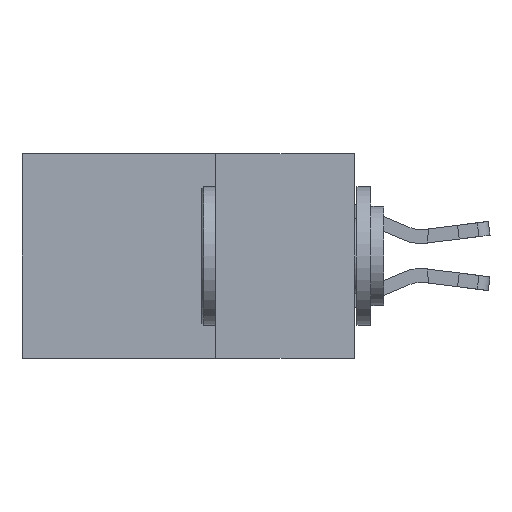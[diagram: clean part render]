
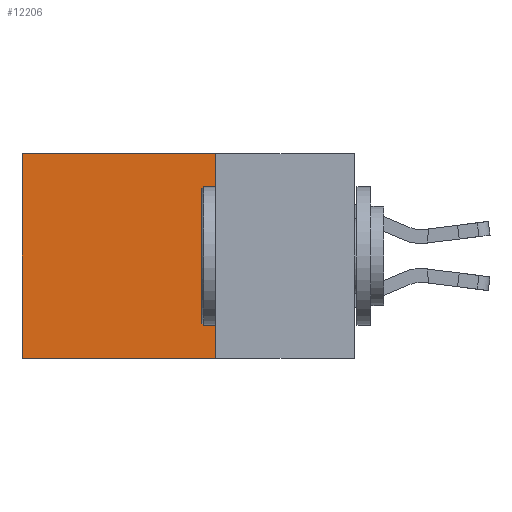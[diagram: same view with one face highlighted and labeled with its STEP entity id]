
A CAD part, left-side view. The second image highlights one B-rep face of the part: STEP entity #12206.
In plain terms, the highlighted planar face has unit normal (-1, 0, 0).
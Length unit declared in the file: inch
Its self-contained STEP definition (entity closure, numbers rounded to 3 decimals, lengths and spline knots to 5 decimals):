
#450 = CARTESIAN_POINT ( 'NONE',  ( 0.298, 0.25, -0.37 ) ) ;
#721 = LINE ( 'NONE', #5988, #22246 ) ;
#822 = FACE_OUTER_BOUND ( 'NONE', #4465, .T. ) ;
#1691 = VERTEX_POINT ( 'NONE', #450 ) ;
#1714 = CARTESIAN_POINT ( 'NONE',  ( 0.298, 0.25, 0. ) ) ;
#2343 = EDGE_CURVE ( 'NONE', #9632, #1691, #10190, .T. ) ;
#3218 = VECTOR ( 'NONE', #13958, 39.37008 ) ;
#3493 = ORIENTED_EDGE ( 'NONE', *, *, #18894, .F. ) ;
#4465 = EDGE_LOOP ( 'NONE', ( #7486, #3493, #18065, #21008 ) ) ;
#4729 = PLANE ( 'NONE',  #17733 ) ;
#4945 = DIRECTION ( 'NONE',  ( 0., 0., -1. ) ) ;
#4955 = LINE ( 'NONE', #19285, #18290 ) ;
#5988 = CARTESIAN_POINT ( 'NONE',  ( 0.298, 0.6, 0. ) ) ;
#7486 = ORIENTED_EDGE ( 'NONE', *, *, #19298, .T. ) ;
#8035 = CARTESIAN_POINT ( 'NONE',  ( 0.298, 0.25, 0. ) ) ;
#8243 = DIRECTION ( 'NONE',  ( 0., 0., -1. ) ) ;
#8584 = CARTESIAN_POINT ( 'NONE',  ( 0.298, 0.25, 0. ) ) ;
#8920 = VERTEX_POINT ( 'NONE', #11416 ) ;
#8934 = DIRECTION ( 'NONE',  ( 0., 1., 0. ) ) ;
#8959 = CARTESIAN_POINT ( 'NONE',  ( 0.298, 0.6, -0.37 ) ) ;
#9628 = VECTOR ( 'NONE', #4945, 39.37008 ) ;
#9632 = VERTEX_POINT ( 'NONE', #8035 ) ;
#9902 = EDGE_CURVE ( 'NONE', #9632, #8920, #12496, .T. ) ;
#10190 = LINE ( 'NONE', #8584, #9628 ) ;
#11416 = CARTESIAN_POINT ( 'NONE',  ( 0.298, 0.6, 0. ) ) ;
#12206 = ADVANCED_FACE ( 'NONE', ( #822 ), #4729, .F. ) ;
#12496 = LINE ( 'NONE', #1714, #3218 ) ;
#13958 = DIRECTION ( 'NONE',  ( 0., 1., 0. ) ) ;
#16906 = CARTESIAN_POINT ( 'NONE',  ( 0.298, 0.25, 0. ) ) ;
#17733 = AXIS2_PLACEMENT_3D ( 'NONE', #16906, #18627, #8243 ) ;
#18065 = ORIENTED_EDGE ( 'NONE', *, *, #2343, .F. ) ;
#18254 = VERTEX_POINT ( 'NONE', #8959 ) ;
#18290 = VECTOR ( 'NONE', #8934, 39.37008 ) ;
#18627 = DIRECTION ( 'NONE',  ( 1., 0., 0. ) ) ;
#18894 = EDGE_CURVE ( 'NONE', #1691, #18254, #4955, .T. ) ;
#19285 = CARTESIAN_POINT ( 'NONE',  ( 0.298, 0.25, -0.37 ) ) ;
#19298 = EDGE_CURVE ( 'NONE', #8920, #18254, #721, .T. ) ;
#19854 = DIRECTION ( 'NONE',  ( 0., 0., -1. ) ) ;
#21008 = ORIENTED_EDGE ( 'NONE', *, *, #9902, .T. ) ;
#22246 = VECTOR ( 'NONE', #19854, 39.37008 ) ;
